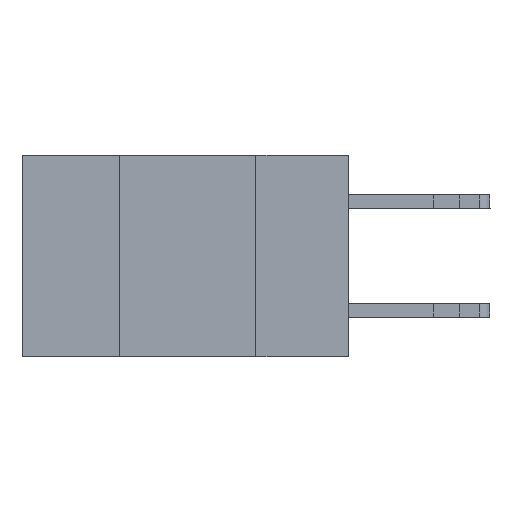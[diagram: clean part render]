
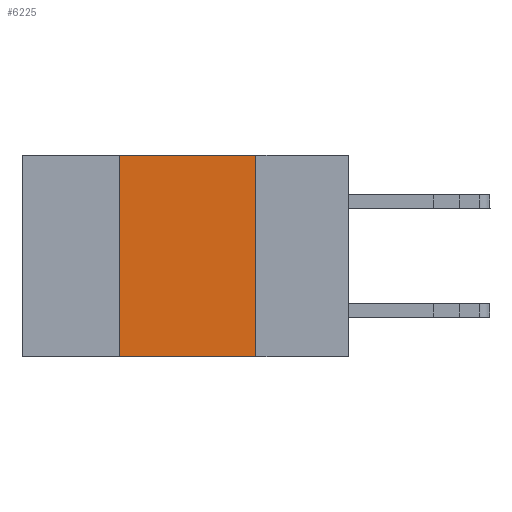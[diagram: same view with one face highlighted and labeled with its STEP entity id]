
A CAD part, left-side view. The second image highlights one B-rep face of the part: STEP entity #6225.
In plain terms, the highlighted planar face has unit normal (-1, 0, 0).
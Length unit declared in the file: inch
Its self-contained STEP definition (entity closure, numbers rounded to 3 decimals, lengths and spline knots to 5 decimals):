
#74 = VECTOR ( 'NONE', #5926, 39.37008 ) ;
#166 = VECTOR ( 'NONE', #5272, 39.37008 ) ;
#1700 = EDGE_CURVE ( 'NONE', #2671, #6638, #9282, .T. ) ;
#1729 = PLANE ( 'NONE',  #5380 ) ;
#2250 = ORIENTED_EDGE ( 'NONE', *, *, #8261, .F. ) ;
#2671 = VERTEX_POINT ( 'NONE', #5362 ) ;
#2758 = CARTESIAN_POINT ( 'NONE',  ( 0., 0.42, 0. ) ) ;
#3493 = CARTESIAN_POINT ( 'NONE',  ( 0., 0.17, -0.37 ) ) ;
#4202 = CARTESIAN_POINT ( 'NONE',  ( 0., 0.17, -0.37 ) ) ;
#4469 = EDGE_CURVE ( 'NONE', #11097, #7226, #11190, .T. ) ;
#4739 = DIRECTION ( 'NONE',  ( 0., 0., -1. ) ) ;
#4999 = ORIENTED_EDGE ( 'NONE', *, *, #1700, .T. ) ;
#5154 = ORIENTED_EDGE ( 'NONE', *, *, #7442, .F. ) ;
#5248 = VECTOR ( 'NONE', #6444, 39.37008 ) ;
#5272 = DIRECTION ( 'NONE',  ( 0., 0., -1. ) ) ;
#5362 = CARTESIAN_POINT ( 'NONE',  ( 0., 0.42, -0.37 ) ) ;
#5380 = AXIS2_PLACEMENT_3D ( 'NONE', #11120, #11295, #4739 ) ;
#5926 = DIRECTION ( 'NONE',  ( 0., 0., 1. ) ) ;
#6225 = ADVANCED_FACE ( 'NONE', ( #6508 ), #1729, .F. ) ;
#6444 = DIRECTION ( 'NONE',  ( 0., -1., 0. ) ) ;
#6508 = FACE_OUTER_BOUND ( 'NONE', #11757, .T. ) ;
#6571 = CARTESIAN_POINT ( 'NONE',  ( 0., 0.6, 0. ) ) ;
#6638 = VERTEX_POINT ( 'NONE', #4202 ) ;
#6844 = CARTESIAN_POINT ( 'NONE',  ( 0., 0.42, -0.37 ) ) ;
#7226 = VERTEX_POINT ( 'NONE', #9356 ) ;
#7442 = EDGE_CURVE ( 'NONE', #7226, #6638, #11935, .T. ) ;
#8261 = EDGE_CURVE ( 'NONE', #2671, #11097, #10527, .T. ) ;
#9282 = LINE ( 'NONE', #9393, #5248 ) ;
#9356 = CARTESIAN_POINT ( 'NONE',  ( 0., 0.17, 0. ) ) ;
#9393 = CARTESIAN_POINT ( 'NONE',  ( 0., 0.6, -0.37 ) ) ;
#9469 = DIRECTION ( 'NONE',  ( 0., -1., 0. ) ) ;
#9933 = ORIENTED_EDGE ( 'NONE', *, *, #4469, .F. ) ;
#10527 = LINE ( 'NONE', #6844, #74 ) ;
#10841 = VECTOR ( 'NONE', #9469, 39.37008 ) ;
#11097 = VERTEX_POINT ( 'NONE', #2758 ) ;
#11120 = CARTESIAN_POINT ( 'NONE',  ( 0., 0.6, 0. ) ) ;
#11190 = LINE ( 'NONE', #6571, #10841 ) ;
#11295 = DIRECTION ( 'NONE',  ( 1., 0., 0. ) ) ;
#11757 = EDGE_LOOP ( 'NONE', ( #5154, #9933, #2250, #4999 ) ) ;
#11935 = LINE ( 'NONE', #3493, #166 ) ;
